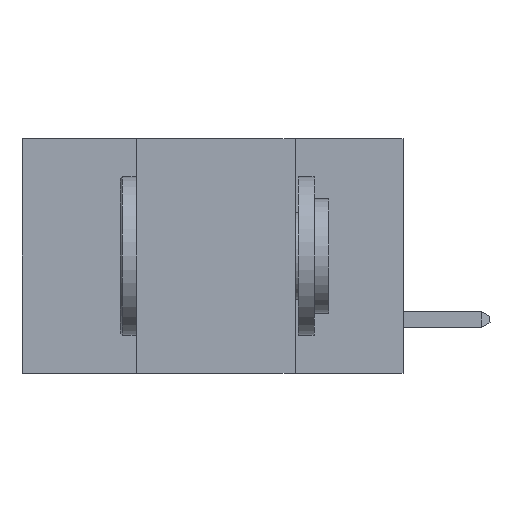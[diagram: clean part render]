
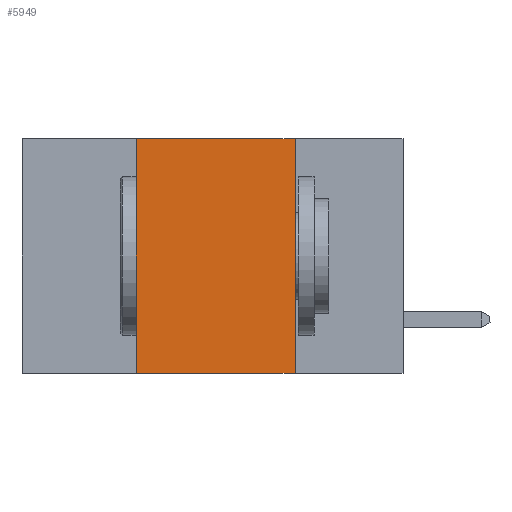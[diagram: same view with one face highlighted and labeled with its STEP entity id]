
A CAD part, left-side view. The second image highlights one B-rep face of the part: STEP entity #5949.
In plain terms, the highlighted planar face has unit normal (-1, 0, 0).
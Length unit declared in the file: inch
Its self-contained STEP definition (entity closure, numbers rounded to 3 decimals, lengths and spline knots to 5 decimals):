
#302 = DIRECTION ( 'NONE',  ( 1., 0., 0. ) ) ;
#470 = CARTESIAN_POINT ( 'NONE',  ( 0., 0.6, 0. ) ) ;
#472 = CARTESIAN_POINT ( 'NONE',  ( 0., 0.17, 0. ) ) ;
#601 = CARTESIAN_POINT ( 'NONE',  ( 0., 0.6, 0. ) ) ;
#1084 = LINE ( 'NONE', #472, #12453 ) ;
#1248 = DIRECTION ( 'NONE',  ( 0., 0., 1. ) ) ;
#1769 = DIRECTION ( 'NONE',  ( 0., -1., 0. ) ) ;
#2052 = VECTOR ( 'NONE', #1769, 39.37008 ) ;
#2223 = EDGE_CURVE ( 'NONE', #3766, #8898, #1084, .T. ) ;
#2499 = PLANE ( 'NONE',  #10987 ) ;
#2606 = EDGE_CURVE ( 'NONE', #11588, #9601, #5734, .T. ) ;
#2656 = EDGE_CURVE ( 'NONE', #11588, #8898, #10468, .T. ) ;
#3732 = EDGE_LOOP ( 'NONE', ( #4104, #8504, #4838, #10852 ) ) ;
#3766 = VERTEX_POINT ( 'NONE', #5937 ) ;
#4104 = ORIENTED_EDGE ( 'NONE', *, *, #2223, .F. ) ;
#4838 = ORIENTED_EDGE ( 'NONE', *, *, #2606, .F. ) ;
#5734 = LINE ( 'NONE', #6445, #11083 ) ;
#5937 = CARTESIAN_POINT ( 'NONE',  ( 0., 0.17, 0. ) ) ;
#5949 = ADVANCED_FACE ( 'NONE', ( #9263 ), #2499, .F. ) ;
#6445 = CARTESIAN_POINT ( 'NONE',  ( 0., 0.42, 0. ) ) ;
#8504 = ORIENTED_EDGE ( 'NONE', *, *, #14022, .F. ) ;
#8898 = VERTEX_POINT ( 'NONE', #12731 ) ;
#9072 = CARTESIAN_POINT ( 'NONE',  ( 0., 0.42, 0. ) ) ;
#9127 = CARTESIAN_POINT ( 'NONE',  ( 0., 0.42, -0.37 ) ) ;
#9263 = FACE_OUTER_BOUND ( 'NONE', #3732, .T. ) ;
#9601 = VERTEX_POINT ( 'NONE', #9072 ) ;
#10468 = LINE ( 'NONE', #10588, #13394 ) ;
#10588 = CARTESIAN_POINT ( 'NONE',  ( 0., 0.6, -0.37 ) ) ;
#10852 = ORIENTED_EDGE ( 'NONE', *, *, #2656, .T. ) ;
#10987 = AXIS2_PLACEMENT_3D ( 'NONE', #601, #302, #14341 ) ;
#11083 = VECTOR ( 'NONE', #1248, 39.37008 ) ;
#11512 = LINE ( 'NONE', #470, #2052 ) ;
#11588 = VERTEX_POINT ( 'NONE', #9127 ) ;
#12431 = DIRECTION ( 'NONE',  ( 0., -1., 0. ) ) ;
#12453 = VECTOR ( 'NONE', #13045, 39.37008 ) ;
#12731 = CARTESIAN_POINT ( 'NONE',  ( 0., 0.17, -0.37 ) ) ;
#13045 = DIRECTION ( 'NONE',  ( 0., 0., -1. ) ) ;
#13394 = VECTOR ( 'NONE', #12431, 39.37008 ) ;
#14022 = EDGE_CURVE ( 'NONE', #9601, #3766, #11512, .T. ) ;
#14341 = DIRECTION ( 'NONE',  ( 0., 0., -1. ) ) ;
